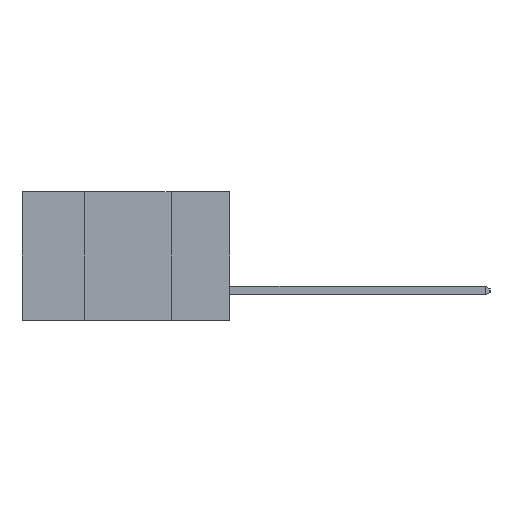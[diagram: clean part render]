
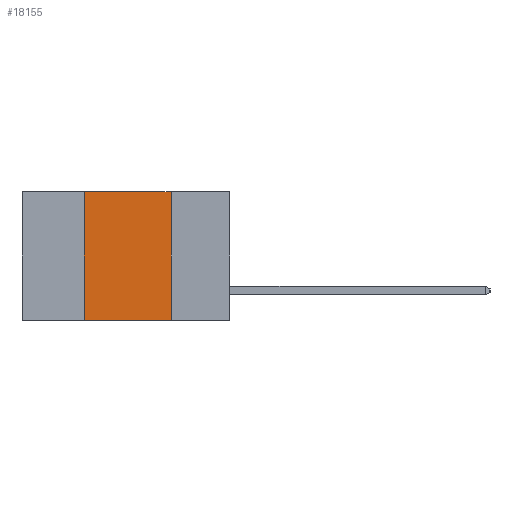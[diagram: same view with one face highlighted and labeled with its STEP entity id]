
A CAD part, left-side view. The second image highlights one B-rep face of the part: STEP entity #18155.
In plain terms, the highlighted planar face has unit normal (-1, 0, 0).
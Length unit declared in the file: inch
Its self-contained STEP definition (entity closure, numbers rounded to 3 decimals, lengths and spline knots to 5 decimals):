
#626 = VERTEX_POINT ( 'NONE', #24687 ) ;
#1287 = DIRECTION ( 'NONE',  ( 0., 0., 1. ) ) ;
#1994 = ORIENTED_EDGE ( 'NONE', *, *, #14380, .F. ) ;
#2105 = VERTEX_POINT ( 'NONE', #6890 ) ;
#2566 = CARTESIAN_POINT ( 'NONE',  ( 0., 0.42, 0. ) ) ;
#2583 = VECTOR ( 'NONE', #1287, 39.37008 ) ;
#4128 = LINE ( 'NONE', #6595, #24487 ) ;
#4449 = LINE ( 'NONE', #19138, #24768 ) ;
#6294 = AXIS2_PLACEMENT_3D ( 'NONE', #16050, #8001, #21719 ) ;
#6483 = CARTESIAN_POINT ( 'NONE',  ( 0., 0.17, 0. ) ) ;
#6491 = LINE ( 'NONE', #24159, #11987 ) ;
#6595 = CARTESIAN_POINT ( 'NONE',  ( 0., 0.17, 0. ) ) ;
#6890 = CARTESIAN_POINT ( 'NONE',  ( 0., 0.42, -0.37 ) ) ;
#8001 = DIRECTION ( 'NONE',  ( 1., 0., 0. ) ) ;
#8090 = LINE ( 'NONE', #17528, #2583 ) ;
#10806 = EDGE_CURVE ( 'NONE', #15013, #626, #4128, .T. ) ;
#11006 = EDGE_CURVE ( 'NONE', #2105, #626, #4449, .T. ) ;
#11987 = VECTOR ( 'NONE', #12727, 39.37008 ) ;
#12319 = ORIENTED_EDGE ( 'NONE', *, *, #10806, .F. ) ;
#12727 = DIRECTION ( 'NONE',  ( 0., -1., 0. ) ) ;
#12799 = DIRECTION ( 'NONE',  ( 0., 0., -1. ) ) ;
#14380 = EDGE_CURVE ( 'NONE', #19719, #15013, #6491, .T. ) ;
#15013 = VERTEX_POINT ( 'NONE', #6483 ) ;
#15154 = ORIENTED_EDGE ( 'NONE', *, *, #19956, .F. ) ;
#16050 = CARTESIAN_POINT ( 'NONE',  ( 0., 0.6, 0. ) ) ;
#16767 = FACE_OUTER_BOUND ( 'NONE', #25533, .T. ) ;
#17528 = CARTESIAN_POINT ( 'NONE',  ( 0., 0.42, 0. ) ) ;
#18155 = ADVANCED_FACE ( 'NONE', ( #16767 ), #19845, .F. ) ;
#19138 = CARTESIAN_POINT ( 'NONE',  ( 0., 0.6, -0.37 ) ) ;
#19719 = VERTEX_POINT ( 'NONE', #2566 ) ;
#19845 = PLANE ( 'NONE',  #6294 ) ;
#19956 = EDGE_CURVE ( 'NONE', #2105, #19719, #8090, .T. ) ;
#21719 = DIRECTION ( 'NONE',  ( 0., 0., -1. ) ) ;
#24159 = CARTESIAN_POINT ( 'NONE',  ( 0., 0.6, 0. ) ) ;
#24329 = ORIENTED_EDGE ( 'NONE', *, *, #11006, .T. ) ;
#24487 = VECTOR ( 'NONE', #12799, 39.37008 ) ;
#24687 = CARTESIAN_POINT ( 'NONE',  ( 0., 0.17, -0.37 ) ) ;
#24768 = VECTOR ( 'NONE', #24790, 39.37008 ) ;
#24790 = DIRECTION ( 'NONE',  ( 0., -1., 0. ) ) ;
#25533 = EDGE_LOOP ( 'NONE', ( #12319, #1994, #15154, #24329 ) ) ;
